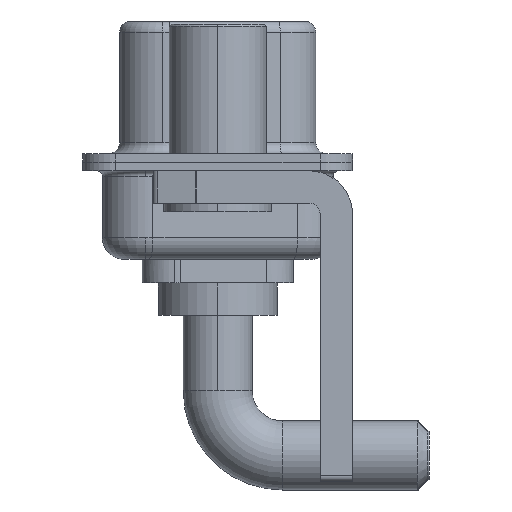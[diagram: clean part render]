
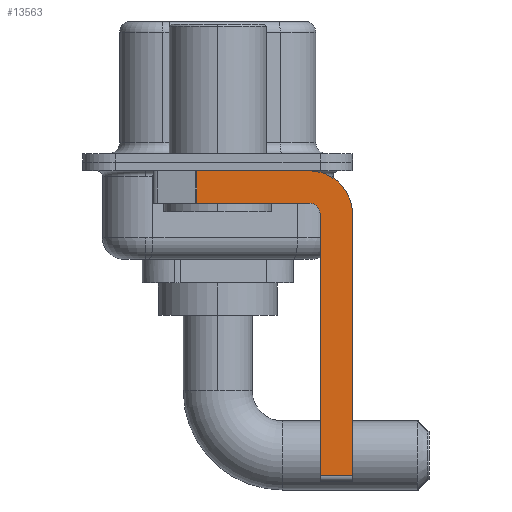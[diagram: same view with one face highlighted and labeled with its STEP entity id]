
A CAD part, left-side view. The second image highlights one B-rep face of the part: STEP entity #13563.
In plain terms, the highlighted planar face has unit normal (-1, 0, 0).
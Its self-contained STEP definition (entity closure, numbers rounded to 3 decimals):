
#384 = DIRECTION ( 'NONE',  ( 1., 0., 0. ) ) ;
#767 = CARTESIAN_POINT ( 'NONE',  ( -2.9, -6.25, -14.55 ) ) ;
#996 = LINE ( 'NONE', #8519, #14976 ) ;
#1103 = LINE ( 'NONE', #6347, #5246 ) ;
#1323 = CARTESIAN_POINT ( 'NONE',  ( -2.9, 0.978, -0.4 ) ) ;
#1402 = FACE_OUTER_BOUND ( 'NONE', #13721, .T. ) ;
#1593 = EDGE_CURVE ( 'NONE', #16290, #6169, #10498, .T. ) ;
#1661 = PLANE ( 'NONE',  #9140 ) ;
#1982 = CARTESIAN_POINT ( 'NONE',  ( -2.9, -4.25, -2.4 ) ) ;
#2378 = EDGE_CURVE ( 'NONE', #10742, #8158, #1103, .T. ) ;
#2651 = ORIENTED_EDGE ( 'NONE', *, *, #5945, .T. ) ;
#2798 = DIRECTION ( 'NONE',  ( -1., 0., 0. ) ) ;
#3044 = LINE ( 'NONE', #13763, #8710 ) ;
#3721 = EDGE_CURVE ( 'NONE', #11757, #7288, #3044, .T. ) ;
#3795 = VERTEX_POINT ( 'NONE', #12818 ) ;
#5045 = VERTEX_POINT ( 'NONE', #14517 ) ;
#5246 = VECTOR ( 'NONE', #15183, 1000. ) ;
#5308 = AXIS2_PLACEMENT_3D ( 'NONE', #1982, #8730, #12456 ) ;
#5696 = CARTESIAN_POINT ( 'NONE',  ( -2.9, -4.25, -1.9 ) ) ;
#5724 = ORIENTED_EDGE ( 'NONE', *, *, #12583, .F. ) ;
#5945 = EDGE_CURVE ( 'NONE', #11757, #5045, #996, .T. ) ;
#6108 = LINE ( 'NONE', #16750, #15047 ) ;
#6169 = VERTEX_POINT ( 'NONE', #5696 ) ;
#6347 = CARTESIAN_POINT ( 'NONE',  ( -2.9, -6.25, -2.4 ) ) ;
#6662 = CARTESIAN_POINT ( 'NONE',  ( -2.9, -4.25, -2.4 ) ) ;
#6742 = DIRECTION ( 'NONE',  ( 0., 0., 1. ) ) ;
#7288 = VERTEX_POINT ( 'NONE', #11238 ) ;
#7485 = DIRECTION ( 'NONE',  ( 0., -1., 0. ) ) ;
#8158 = VERTEX_POINT ( 'NONE', #767 ) ;
#8519 = CARTESIAN_POINT ( 'NONE',  ( -2.9, 0.978, -1.9 ) ) ;
#8642 = DIRECTION ( 'NONE',  ( 0., 0., 1. ) ) ;
#8710 = VECTOR ( 'NONE', #10956, 1000. ) ;
#8730 = DIRECTION ( 'NONE',  ( 1., 0., 0. ) ) ;
#8867 = VECTOR ( 'NONE', #8642, 1000. ) ;
#9140 = AXIS2_PLACEMENT_3D ( 'NONE', #9263, #384, #13084 ) ;
#9152 = EDGE_CURVE ( 'NONE', #6169, #5045, #16051, .T. ) ;
#9263 = CARTESIAN_POINT ( 'NONE',  ( -2.9, -4.25, -2.4 ) ) ;
#9875 = VECTOR ( 'NONE', #15011, 1000. ) ;
#10156 = CARTESIAN_POINT ( 'NONE',  ( -2.9, -6.25, -2.4 ) ) ;
#10220 = AXIS2_PLACEMENT_3D ( 'NONE', #6662, #2798, #6742 ) ;
#10231 = ORIENTED_EDGE ( 'NONE', *, *, #9152, .F. ) ;
#10498 = CIRCLE ( 'NONE', #10220, 0.5 ) ;
#10742 = VERTEX_POINT ( 'NONE', #10156 ) ;
#10827 = ORIENTED_EDGE ( 'NONE', *, *, #11206, .T. ) ;
#10956 = DIRECTION ( 'NONE',  ( 0., -1., 0. ) ) ;
#11206 = EDGE_CURVE ( 'NONE', #3795, #8158, #6108, .T. ) ;
#11238 = CARTESIAN_POINT ( 'NONE',  ( -2.9, -4.25, -0.4 ) ) ;
#11501 = ORIENTED_EDGE ( 'NONE', *, *, #16863, .F. ) ;
#11757 = VERTEX_POINT ( 'NONE', #1323 ) ;
#12456 = DIRECTION ( 'NONE',  ( 0., 0., -1. ) ) ;
#12533 = LINE ( 'NONE', #13910, #8867 ) ;
#12583 = EDGE_CURVE ( 'NONE', #7288, #10742, #12913, .T. ) ;
#12818 = CARTESIAN_POINT ( 'NONE',  ( -2.9, -4.75, -14.55 ) ) ;
#12913 = CIRCLE ( 'NONE', #5308, 2. ) ;
#13084 = DIRECTION ( 'NONE',  ( 0., 0., -1. ) ) ;
#13563 = ADVANCED_FACE ( 'NONE', ( #1402 ), #1661, .F. ) ;
#13708 = DIRECTION ( 'NONE',  ( 0., 0., -1. ) ) ;
#13721 = EDGE_LOOP ( 'NONE', ( #15754, #2651, #10231, #15315, #11501, #10827, #15631, #5724 ) ) ;
#13763 = CARTESIAN_POINT ( 'NONE',  ( -2.9, 3., -0.4 ) ) ;
#13910 = CARTESIAN_POINT ( 'NONE',  ( -2.9, -4.75, -14.8 ) ) ;
#14147 = CARTESIAN_POINT ( 'NONE',  ( -2.9, -4.75, -2.4 ) ) ;
#14517 = CARTESIAN_POINT ( 'NONE',  ( -2.9, 0.978, -1.9 ) ) ;
#14976 = VECTOR ( 'NONE', #13708, 1000. ) ;
#15011 = DIRECTION ( 'NONE',  ( 0., 1., 0. ) ) ;
#15047 = VECTOR ( 'NONE', #7485, 1000. ) ;
#15183 = DIRECTION ( 'NONE',  ( 0., 0., -1. ) ) ;
#15315 = ORIENTED_EDGE ( 'NONE', *, *, #1593, .F. ) ;
#15631 = ORIENTED_EDGE ( 'NONE', *, *, #2378, .F. ) ;
#15754 = ORIENTED_EDGE ( 'NONE', *, *, #3721, .F. ) ;
#15972 = CARTESIAN_POINT ( 'NONE',  ( -2.9, -4.25, -1.9 ) ) ;
#16051 = LINE ( 'NONE', #15972, #9875 ) ;
#16290 = VERTEX_POINT ( 'NONE', #14147 ) ;
#16750 = CARTESIAN_POINT ( 'NONE',  ( -2.9, -4.25, -14.55 ) ) ;
#16863 = EDGE_CURVE ( 'NONE', #3795, #16290, #12533, .T. ) ;
